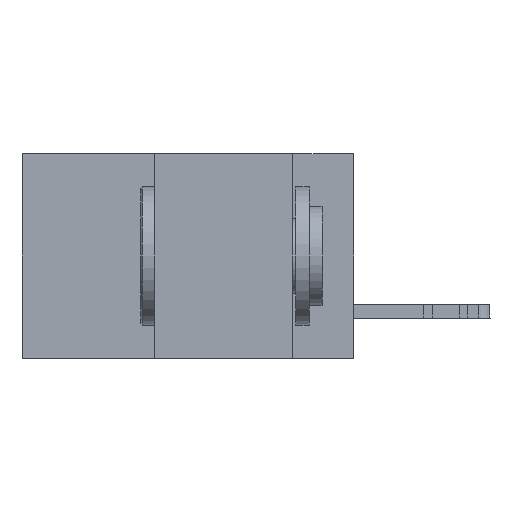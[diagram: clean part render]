
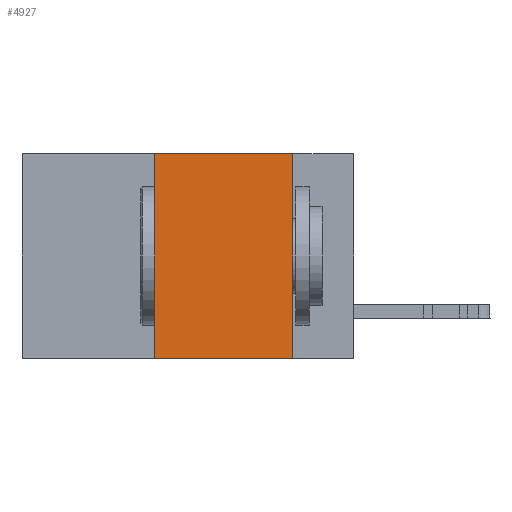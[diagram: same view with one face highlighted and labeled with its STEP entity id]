
A CAD part, left-side view. The second image highlights one B-rep face of the part: STEP entity #4927.
In plain terms, the highlighted planar face has unit normal (-1, 0, 0).
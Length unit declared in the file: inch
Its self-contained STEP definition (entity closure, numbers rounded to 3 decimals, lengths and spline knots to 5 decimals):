
#361 = FACE_OUTER_BOUND ( 'NONE', #41090, .T. ) ;
#594 = VERTEX_POINT ( 'NONE', #35550 ) ;
#1633 = VECTOR ( 'NONE', #2008, 39.37008 ) ;
#1636 = LINE ( 'NONE', #29863, #5654 ) ;
#1841 = DIRECTION ( 'NONE',  ( 0., -1., 0. ) ) ;
#1993 = VERTEX_POINT ( 'NONE', #4590 ) ;
#2007 = VERTEX_POINT ( 'NONE', #4381 ) ;
#2008 = DIRECTION ( 'NONE',  ( 0., -1., 0. ) ) ;
#2045 = EDGE_CURVE ( 'NONE', #29437, #1993, #1636, .T. ) ;
#2780 = CARTESIAN_POINT ( 'NONE',  ( 0., 0.36, 0. ) ) ;
#3922 = CARTESIAN_POINT ( 'NONE',  ( 0., 0.11, 0. ) ) ;
#3969 = EDGE_CURVE ( 'NONE', #594, #2007, #8326, .T. ) ;
#4381 = CARTESIAN_POINT ( 'NONE',  ( 0., 0.11, 0. ) ) ;
#4590 = CARTESIAN_POINT ( 'NONE',  ( 0., 0.11, -0.37 ) ) ;
#4927 = ADVANCED_FACE ( 'NONE', ( #361 ), #16815, .F. ) ;
#5654 = VECTOR ( 'NONE', #1841, 39.37008 ) ;
#7103 = DIRECTION ( 'NONE',  ( 0., 0., -1. ) ) ;
#7322 = DIRECTION ( 'NONE',  ( 1., 0., 0. ) ) ;
#8326 = LINE ( 'NONE', #37176, #1633 ) ;
#9174 = AXIS2_PLACEMENT_3D ( 'NONE', #37910, #7322, #7103 ) ;
#11149 = EDGE_CURVE ( 'NONE', #29437, #594, #40905, .T. ) ;
#15794 = ORIENTED_EDGE ( 'NONE', *, *, #2045, .T. ) ;
#16323 = EDGE_CURVE ( 'NONE', #2007, #1993, #22911, .T. ) ;
#16793 = CARTESIAN_POINT ( 'NONE',  ( 0., 0.36, -0.37 ) ) ;
#16815 = PLANE ( 'NONE',  #9174 ) ;
#19097 = ORIENTED_EDGE ( 'NONE', *, *, #11149, .F. ) ;
#20813 = ORIENTED_EDGE ( 'NONE', *, *, #16323, .F. ) ;
#22193 = DIRECTION ( 'NONE',  ( 0., 0., 1. ) ) ;
#22691 = DIRECTION ( 'NONE',  ( 0., 0., -1. ) ) ;
#22911 = LINE ( 'NONE', #3922, #28461 ) ;
#28124 = ORIENTED_EDGE ( 'NONE', *, *, #3969, .F. ) ;
#28461 = VECTOR ( 'NONE', #22691, 39.37008 ) ;
#29437 = VERTEX_POINT ( 'NONE', #16793 ) ;
#29863 = CARTESIAN_POINT ( 'NONE',  ( 0., 0.6, -0.37 ) ) ;
#35550 = CARTESIAN_POINT ( 'NONE',  ( 0., 0.36, 0. ) ) ;
#36883 = VECTOR ( 'NONE', #22193, 39.37008 ) ;
#37176 = CARTESIAN_POINT ( 'NONE',  ( 0., 0.6, 0. ) ) ;
#37910 = CARTESIAN_POINT ( 'NONE',  ( 0., 0.6, 0. ) ) ;
#40905 = LINE ( 'NONE', #2780, #36883 ) ;
#41090 = EDGE_LOOP ( 'NONE', ( #20813, #28124, #19097, #15794 ) ) ;
